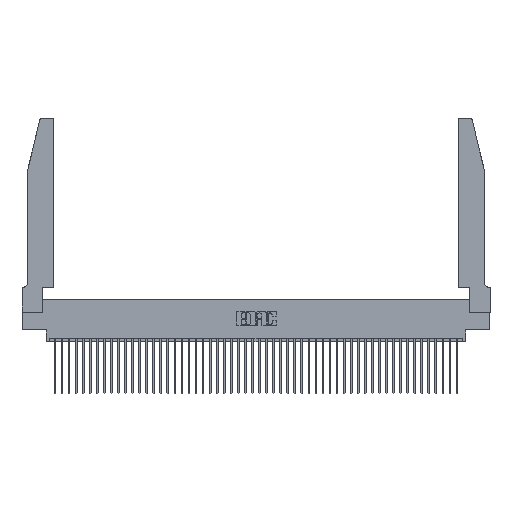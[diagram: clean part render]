
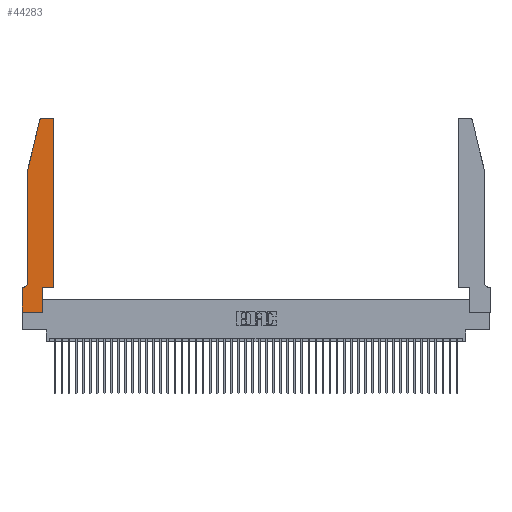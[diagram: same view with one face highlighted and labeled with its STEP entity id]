
A CAD part, top view. The second image highlights one B-rep face of the part: STEP entity #44283.
In plain terms, the highlighted planar face has unit normal (0, 0, 1).
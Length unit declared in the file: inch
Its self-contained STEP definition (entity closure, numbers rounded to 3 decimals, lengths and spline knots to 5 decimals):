
#1353 = VERTEX_POINT ( 'NONE', #13136 ) ;
#1607 = VERTEX_POINT ( 'NONE', #33171 ) ;
#2053 = VECTOR ( 'NONE', #43346, 39.37008 ) ;
#2408 = CARTESIAN_POINT ( 'NONE',  ( 0.4505, 0.35, 0.37 ) ) ;
#2429 = CARTESIAN_POINT ( 'NONE',  ( 0., 0., 0.37 ) ) ;
#2511 = VERTEX_POINT ( 'NONE', #5635 ) ;
#4056 = DIRECTION ( 'NONE',  ( -1., 0., 0. ) ) ;
#4476 = EDGE_CURVE ( 'NONE', #30751, #12998, #4518, .T. ) ;
#4518 = LINE ( 'NONE', #8048, #25634 ) ;
#5160 = CARTESIAN_POINT ( 'NONE',  ( 0.284, 2.75, 0.37 ) ) ;
#5415 = AXIS2_PLACEMENT_3D ( 'NONE', #39604, #17359, #43315 ) ;
#5435 = ORIENTED_EDGE ( 'NONE', *, *, #11029, .T. ) ;
#5577 = LINE ( 'NONE', #2429, #42884 ) ;
#5635 = CARTESIAN_POINT ( 'NONE',  ( 0.0755, 0.42, 0.37 ) ) ;
#5734 = CARTESIAN_POINT ( 'NONE',  ( 0.0755, 2., 0.37 ) ) ;
#7448 = LINE ( 'NONE', #43278, #9794 ) ;
#8048 = CARTESIAN_POINT ( 'NONE',  ( 0., 0., 0.37 ) ) ;
#8311 = ORIENTED_EDGE ( 'NONE', *, *, #37940, .T. ) ;
#9304 = ORIENTED_EDGE ( 'NONE', *, *, #4476, .T. ) ;
#9515 = EDGE_CURVE ( 'NONE', #13574, #20705, #28999, .T. ) ;
#9582 = VECTOR ( 'NONE', #22428, 39.37008 ) ;
#9794 = VECTOR ( 'NONE', #46966, 39.37008 ) ;
#10296 = CARTESIAN_POINT ( 'NONE',  ( 0.4505, 0.35, 0.37 ) ) ;
#11029 = EDGE_CURVE ( 'NONE', #20705, #18920, #18430, .T. ) ;
#11828 = DIRECTION ( 'NONE',  ( 0., -1., 0. ) ) ;
#11870 = ORIENTED_EDGE ( 'NONE', *, *, #22860, .T. ) ;
#12015 = LINE ( 'NONE', #5734, #39394 ) ;
#12434 = EDGE_LOOP ( 'NONE', ( #28312, #5435, #8311, #32045, #26786, #32235, #9304, #15099, #11870, #36808, #31001, #44258 ) ) ;
#12670 = CARTESIAN_POINT ( 'NONE',  ( 0.0755, 2., 0.37 ) ) ;
#12998 = VERTEX_POINT ( 'NONE', #21655 ) ;
#13033 = CARTESIAN_POINT ( 'NONE',  ( 0.25487, 2.72718, 0.37 ) ) ;
#13136 = CARTESIAN_POINT ( 'NONE',  ( 0.2865, 0., 0.37 ) ) ;
#13574 = VERTEX_POINT ( 'NONE', #24533 ) ;
#13977 = VECTOR ( 'NONE', #4056, 39.37008 ) ;
#14829 = CARTESIAN_POINT ( 'NONE',  ( 0.284, 2.72, 0.37 ) ) ;
#15099 = ORIENTED_EDGE ( 'NONE', *, *, #44073, .T. ) ;
#15849 = EDGE_CURVE ( 'NONE', #45362, #47500, #29617, .T. ) ;
#16689 = DIRECTION ( 'NONE',  ( 0., 1., 0. ) ) ;
#17359 = DIRECTION ( 'NONE',  ( 0., 0., -1. ) ) ;
#17941 = EDGE_CURVE ( 'NONE', #26267, #30751, #23909, .T. ) ;
#18430 = CIRCLE ( 'NONE', #45916, 0.03 ) ;
#18597 = DIRECTION ( 'NONE',  ( 1., 0., 0. ) ) ;
#18681 = CARTESIAN_POINT ( 'NONE',  ( 0.2865, 0.35, 0.37 ) ) ;
#18704 = DIRECTION ( 'NONE',  ( 0., 0., 1. ) ) ;
#18920 = VERTEX_POINT ( 'NONE', #13033 ) ;
#19018 = DIRECTION ( 'NONE',  ( 0., 0., 1. ) ) ;
#19548 = LINE ( 'NONE', #18681, #9582 ) ;
#20235 = VECTOR ( 'NONE', #40893, 39.37008 ) ;
#20705 = VERTEX_POINT ( 'NONE', #5160 ) ;
#21400 = CIRCLE ( 'NONE', #32552, 0.03 ) ;
#21655 = CARTESIAN_POINT ( 'NONE',  ( 0., 0., 0.37 ) ) ;
#22098 = CARTESIAN_POINT ( 'NONE',  ( 0.2605, 2.75, 0.37 ) ) ;
#22428 = DIRECTION ( 'NONE',  ( 0., 1., 0. ) ) ;
#22860 = EDGE_CURVE ( 'NONE', #1353, #45362, #19548, .T. ) ;
#23909 = LINE ( 'NONE', #44911, #13977 ) ;
#24533 = CARTESIAN_POINT ( 'NONE',  ( 0.4205, 2.75, 0.37 ) ) ;
#25072 = DIRECTION ( 'NONE',  ( 1., 0., 0. ) ) ;
#25634 = VECTOR ( 'NONE', #11828, 39.37008 ) ;
#25731 = VERTEX_POINT ( 'NONE', #12670 ) ;
#26267 = VERTEX_POINT ( 'NONE', #34153 ) ;
#26495 = EDGE_CURVE ( 'NONE', #47500, #1607, #26764, .T. ) ;
#26764 = LINE ( 'NONE', #42670, #36650 ) ;
#26786 = ORIENTED_EDGE ( 'NONE', *, *, #36315, .T. ) ;
#28312 = ORIENTED_EDGE ( 'NONE', *, *, #9515, .T. ) ;
#28999 = LINE ( 'NONE', #22098, #20235 ) ;
#29290 = EDGE_CURVE ( 'NONE', #25731, #2511, #12015, .T. ) ;
#29617 = LINE ( 'NONE', #2408, #2053 ) ;
#30072 = AXIS2_PLACEMENT_3D ( 'NONE', #37223, #18704, #44624 ) ;
#30751 = VERTEX_POINT ( 'NONE', #35198 ) ;
#31001 = ORIENTED_EDGE ( 'NONE', *, *, #26495, .T. ) ;
#31890 = DIRECTION ( 'NONE',  ( 0., -1., 0. ) ) ;
#32045 = ORIENTED_EDGE ( 'NONE', *, *, #29290, .T. ) ;
#32235 = ORIENTED_EDGE ( 'NONE', *, *, #17941, .T. ) ;
#32552 = AXIS2_PLACEMENT_3D ( 'NONE', #41257, #19018, #44923 ) ;
#33171 = CARTESIAN_POINT ( 'NONE',  ( 0.4505, 2.72, 0.37 ) ) ;
#33628 = FACE_OUTER_BOUND ( 'NONE', #12434, .T. ) ;
#34153 = CARTESIAN_POINT ( 'NONE',  ( 0.0055, 0.35, 0.37 ) ) ;
#35198 = CARTESIAN_POINT ( 'NONE',  ( 0., 0.35, 0.37 ) ) ;
#36315 = EDGE_CURVE ( 'NONE', #2511, #26267, #37948, .T. ) ;
#36650 = VECTOR ( 'NONE', #16689, 39.37008 ) ;
#36808 = ORIENTED_EDGE ( 'NONE', *, *, #15849, .T. ) ;
#37223 = CARTESIAN_POINT ( 'NONE',  ( 0., 0.35, 0.37 ) ) ;
#37940 = EDGE_CURVE ( 'NONE', #18920, #25731, #7448, .T. ) ;
#37948 = CIRCLE ( 'NONE', #5415, 0.07 ) ;
#39064 = CARTESIAN_POINT ( 'NONE',  ( 0.2865, 0.35, 0.37 ) ) ;
#39394 = VECTOR ( 'NONE', #31890, 39.37008 ) ;
#39604 = CARTESIAN_POINT ( 'NONE',  ( 0.0055, 0.42, 0.37 ) ) ;
#40822 = DIRECTION ( 'NONE',  ( 0., 0., 1. ) ) ;
#40893 = DIRECTION ( 'NONE',  ( -1., 0., 0. ) ) ;
#41257 = CARTESIAN_POINT ( 'NONE',  ( 0.4205, 2.72, 0.37 ) ) ;
#42670 = CARTESIAN_POINT ( 'NONE',  ( 0.4505, 0.35, 0.37 ) ) ;
#42884 = VECTOR ( 'NONE', #25072, 39.37008 ) ;
#43278 = CARTESIAN_POINT ( 'NONE',  ( 0.0755, 2., 0.37 ) ) ;
#43315 = DIRECTION ( 'NONE',  ( -1., 0., 0. ) ) ;
#43346 = DIRECTION ( 'NONE',  ( 1., 0., 0. ) ) ;
#44073 = EDGE_CURVE ( 'NONE', #12998, #1353, #5577, .T. ) ;
#44258 = ORIENTED_EDGE ( 'NONE', *, *, #44329, .T. ) ;
#44283 = ADVANCED_FACE ( 'NONE', ( #33628 ), #48166, .T. ) ;
#44329 = EDGE_CURVE ( 'NONE', #1607, #13574, #21400, .T. ) ;
#44624 = DIRECTION ( 'NONE',  ( 1., 0., 0. ) ) ;
#44911 = CARTESIAN_POINT ( 'NONE',  ( 0.0755, 0.35, 0.37 ) ) ;
#44923 = DIRECTION ( 'NONE',  ( 1., 0., 0. ) ) ;
#45362 = VERTEX_POINT ( 'NONE', #39064 ) ;
#45916 = AXIS2_PLACEMENT_3D ( 'NONE', #14829, #40822, #18597 ) ;
#46966 = DIRECTION ( 'NONE',  ( -0.239, -0.971, 0. ) ) ;
#47500 = VERTEX_POINT ( 'NONE', #10296 ) ;
#48166 = PLANE ( 'NONE',  #30072 ) ;
